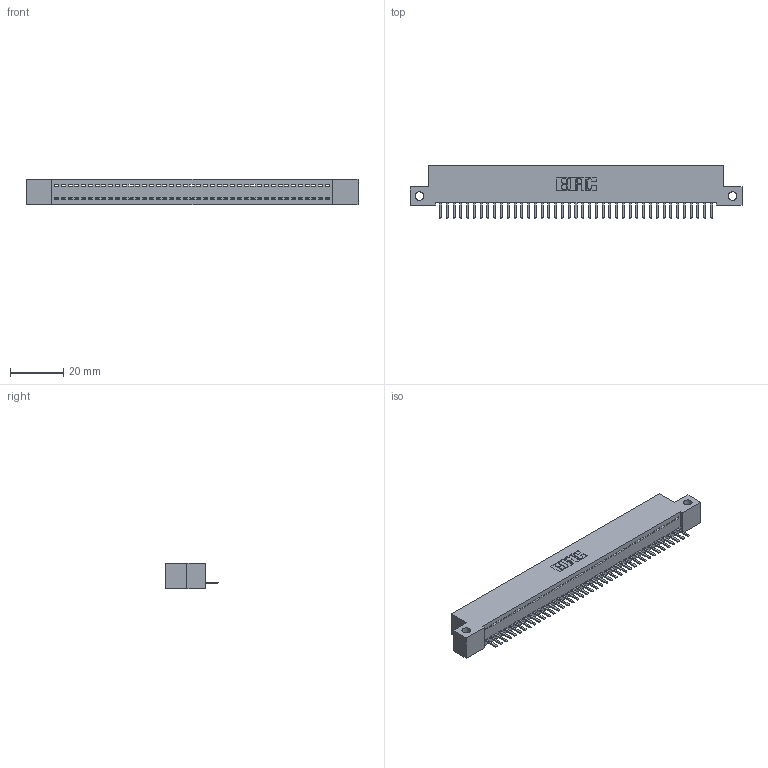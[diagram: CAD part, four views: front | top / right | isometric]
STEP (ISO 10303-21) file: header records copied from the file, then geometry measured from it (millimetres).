
FILE_DESCRIPTION (( 'STEP AP203' ), '1' );
FILE_NAME ('392-041-520-112.STEP', '2019-10-07T20:25:59', ( '' ), ( '' ), 'SwSTEP 2.0', 'SolidWorks 2016', '' );
FILE_SCHEMA (( 'CONFIG_CONTROL_DESIGN' ));
Length unit declared in the file: inch
Products named in the file (3): 342 Part_Side Mount; 345-292-001_345-293-120; 392-041-520-112
Assembly tree (42 placements, depth 2):
  392-041-520-112
    342 Part_Side Mount
    345-292-001_345-293-120  x41
Bounding box: 124.46 x 20.02 x 9.4 mm (x, y, z)
Volume: 10717.1 mm3; surface area: 15178.6 mm2
Topology: 42 solids, 42 shells, 2652 faces, 7843 edges, 5118 vertices
Faces by surface type: plane 1870, cylinder 782
Entity records: 25179 total; most frequent: CARTESIAN_POINT 4361, ORIENTED_EDGE 4326, DIRECTION 3669, EDGE_CURVE 2163, VECTOR 2031, LINE 2031, VERTEX_POINT 1438, AXIS2_PLACEMENT_3D 819
